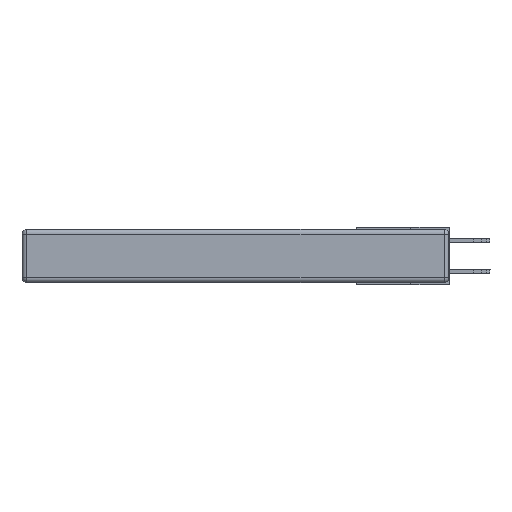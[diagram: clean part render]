
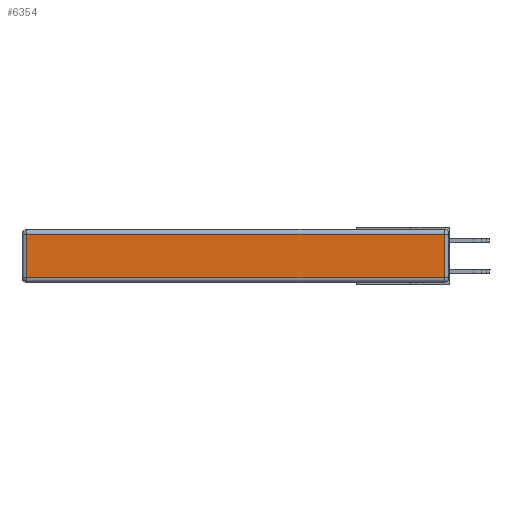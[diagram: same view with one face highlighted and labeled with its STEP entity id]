
A CAD part, left-side view. The second image highlights one B-rep face of the part: STEP entity #6354.
In plain terms, the highlighted planar face has unit normal (-1, 0, 0).
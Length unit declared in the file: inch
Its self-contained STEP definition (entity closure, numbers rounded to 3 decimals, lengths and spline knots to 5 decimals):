
#341 = EDGE_CURVE ( 'NONE', #9722, #8477, #14902, .T. ) ;
#946 = CARTESIAN_POINT ( 'NONE',  ( 0., 2.72, -0.313 ) ) ;
#979 = DIRECTION ( 'NONE',  ( 0., -1., 0. ) ) ;
#995 = EDGE_LOOP ( 'NONE', ( #6877, #7687, #4878, #4550 ) ) ;
#1570 = CARTESIAN_POINT ( 'NONE',  ( 0., 2.75, -0.03 ) ) ;
#1820 = DIRECTION ( 'NONE',  ( 0., 0., 1. ) ) ;
#2189 = LINE ( 'NONE', #13601, #4218 ) ;
#2208 = PLANE ( 'NONE',  #4217 ) ;
#2311 = CARTESIAN_POINT ( 'NONE',  ( 0., 0., -0.343 ) ) ;
#2420 = DIRECTION ( 'NONE',  ( -1., 0., 0. ) ) ;
#3396 = CARTESIAN_POINT ( 'NONE',  ( 0., 0.03, -0.03 ) ) ;
#4211 = VECTOR ( 'NONE', #1820, 39.37008 ) ;
#4217 = AXIS2_PLACEMENT_3D ( 'NONE', #2311, #2420, #5090 ) ;
#4218 = VECTOR ( 'NONE', #7649, 39.37008 ) ;
#4550 = ORIENTED_EDGE ( 'NONE', *, *, #12035, .T. ) ;
#4878 = ORIENTED_EDGE ( 'NONE', *, *, #8244, .T. ) ;
#5021 = FACE_OUTER_BOUND ( 'NONE', #995, .T. ) ;
#5077 = DIRECTION ( 'NONE',  ( 0., 1., 0. ) ) ;
#5090 = DIRECTION ( 'NONE',  ( 0., 0., 1. ) ) ;
#5613 = CARTESIAN_POINT ( 'NONE',  ( 0., 0., -0.313 ) ) ;
#6354 = ADVANCED_FACE ( 'NONE', ( #5021 ), #2208, .T. ) ;
#6877 = ORIENTED_EDGE ( 'NONE', *, *, #12842, .T. ) ;
#7392 = VERTEX_POINT ( 'NONE', #946 ) ;
#7649 = DIRECTION ( 'NONE',  ( 0., 0., -1. ) ) ;
#7687 = ORIENTED_EDGE ( 'NONE', *, *, #341, .T. ) ;
#8244 = EDGE_CURVE ( 'NONE', #8477, #10573, #13935, .T. ) ;
#8477 = VERTEX_POINT ( 'NONE', #3396 ) ;
#9722 = VERTEX_POINT ( 'NONE', #14032 ) ;
#10573 = VERTEX_POINT ( 'NONE', #10864 ) ;
#10864 = CARTESIAN_POINT ( 'NONE',  ( 0., 2.72, -0.03 ) ) ;
#11293 = CARTESIAN_POINT ( 'NONE',  ( 0., 0.03, -0.343 ) ) ;
#12035 = EDGE_CURVE ( 'NONE', #10573, #7392, #2189, .T. ) ;
#12842 = EDGE_CURVE ( 'NONE', #7392, #9722, #13635, .T. ) ;
#13037 = VECTOR ( 'NONE', #5077, 39.37008 ) ;
#13601 = CARTESIAN_POINT ( 'NONE',  ( 0., 2.72, -0.343 ) ) ;
#13635 = LINE ( 'NONE', #5613, #14343 ) ;
#13935 = LINE ( 'NONE', #1570, #13037 ) ;
#14032 = CARTESIAN_POINT ( 'NONE',  ( 0., 0.03, -0.313 ) ) ;
#14343 = VECTOR ( 'NONE', #979, 39.37008 ) ;
#14902 = LINE ( 'NONE', #11293, #4211 ) ;
